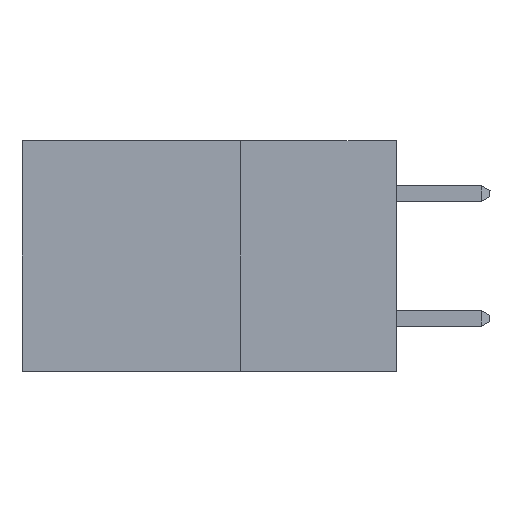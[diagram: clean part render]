
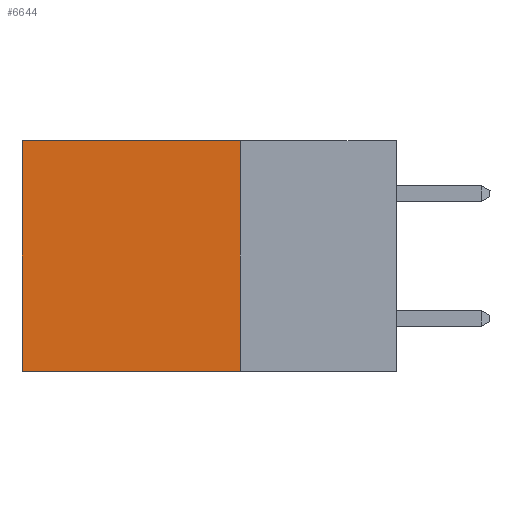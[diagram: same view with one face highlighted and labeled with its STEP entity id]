
A CAD part, left-side view. The second image highlights one B-rep face of the part: STEP entity #6644.
In plain terms, the highlighted planar face has unit normal (-1, 0, 0).
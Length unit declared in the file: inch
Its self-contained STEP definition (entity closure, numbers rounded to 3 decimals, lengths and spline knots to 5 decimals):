
#328 = ORIENTED_EDGE ( 'NONE', *, *, #451, .F. ) ;
#436 = ORIENTED_EDGE ( 'NONE', *, *, #12097, .F. ) ;
#451 = EDGE_CURVE ( 'NONE', #13431, #2441, #13824, .T. ) ;
#691 = CARTESIAN_POINT ( 'NONE',  ( 0.298, 0.25, 0. ) ) ;
#1615 = CARTESIAN_POINT ( 'NONE',  ( 0.298, 0.25, 0. ) ) ;
#1629 = VERTEX_POINT ( 'NONE', #691 ) ;
#1709 = AXIS2_PLACEMENT_3D ( 'NONE', #1615, #15505, #7978 ) ;
#2295 = ORIENTED_EDGE ( 'NONE', *, *, #15527, .T. ) ;
#2440 = LINE ( 'NONE', #5087, #15082 ) ;
#2441 = VERTEX_POINT ( 'NONE', #14482 ) ;
#2900 = PLANE ( 'NONE',  #1709 ) ;
#3738 = VECTOR ( 'NONE', #6964, 39.37008 ) ;
#4788 = DIRECTION ( 'NONE',  ( 0., 0., -1. ) ) ;
#4970 = CARTESIAN_POINT ( 'NONE',  ( 0.298, 0.25, -0.37 ) ) ;
#5016 = EDGE_CURVE ( 'NONE', #9008, #2441, #12703, .T. ) ;
#5087 = CARTESIAN_POINT ( 'NONE',  ( 0.298, 0.25, 0. ) ) ;
#6644 = ADVANCED_FACE ( 'NONE', ( #12479 ), #2900, .F. ) ;
#6964 = DIRECTION ( 'NONE',  ( 0., 1., 0. ) ) ;
#7248 = CARTESIAN_POINT ( 'NONE',  ( 0.298, 0.6, 0. ) ) ;
#7898 = CARTESIAN_POINT ( 'NONE',  ( 0.298, 0.6, 0. ) ) ;
#7978 = DIRECTION ( 'NONE',  ( 0., 0., -1. ) ) ;
#9008 = VERTEX_POINT ( 'NONE', #7898 ) ;
#9258 = EDGE_LOOP ( 'NONE', ( #13006, #328, #436, #2295 ) ) ;
#11001 = CARTESIAN_POINT ( 'NONE',  ( 0.298, 0.25, -0.37 ) ) ;
#12097 = EDGE_CURVE ( 'NONE', #1629, #13431, #12529, .T. ) ;
#12142 = VECTOR ( 'NONE', #14768, 39.37008 ) ;
#12340 = VECTOR ( 'NONE', #4788, 39.37008 ) ;
#12479 = FACE_OUTER_BOUND ( 'NONE', #9258, .T. ) ;
#12529 = LINE ( 'NONE', #13517, #12142 ) ;
#12649 = DIRECTION ( 'NONE',  ( 0., 1., 0. ) ) ;
#12703 = LINE ( 'NONE', #7248, #12340 ) ;
#13006 = ORIENTED_EDGE ( 'NONE', *, *, #5016, .T. ) ;
#13431 = VERTEX_POINT ( 'NONE', #11001 ) ;
#13517 = CARTESIAN_POINT ( 'NONE',  ( 0.298, 0.25, 0. ) ) ;
#13824 = LINE ( 'NONE', #4970, #3738 ) ;
#14482 = CARTESIAN_POINT ( 'NONE',  ( 0.298, 0.6, -0.37 ) ) ;
#14768 = DIRECTION ( 'NONE',  ( 0., 0., -1. ) ) ;
#15082 = VECTOR ( 'NONE', #12649, 39.37008 ) ;
#15505 = DIRECTION ( 'NONE',  ( 1., 0., 0. ) ) ;
#15527 = EDGE_CURVE ( 'NONE', #1629, #9008, #2440, .T. ) ;
